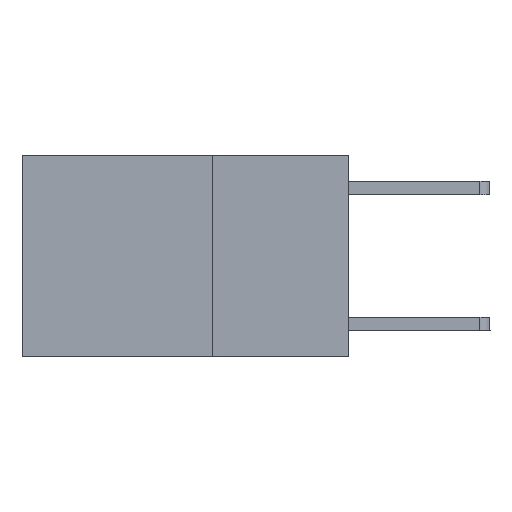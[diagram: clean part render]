
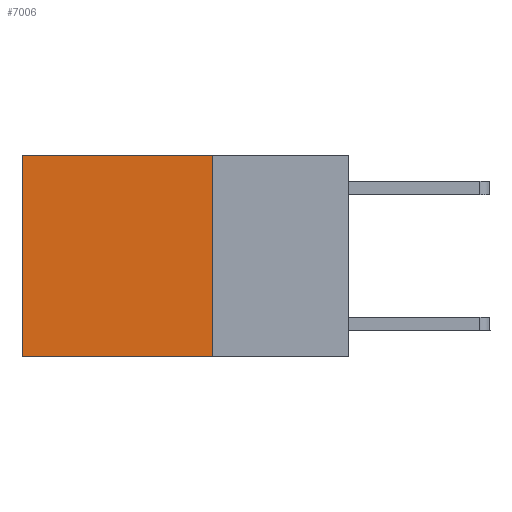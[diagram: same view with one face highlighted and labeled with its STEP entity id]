
A CAD part, left-side view. The second image highlights one B-rep face of the part: STEP entity #7006.
In plain terms, the highlighted planar face has unit normal (-1, 0, 0).
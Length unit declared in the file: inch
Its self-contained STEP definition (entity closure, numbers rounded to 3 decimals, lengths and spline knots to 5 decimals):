
#231 = EDGE_CURVE ( 'NONE', #5409, #7527, #5447, .T. ) ;
#343 = EDGE_CURVE ( 'NONE', #8316, #1577, #7993, .T. ) ;
#571 = ORIENTED_EDGE ( 'NONE', *, *, #9104, .T. ) ;
#599 = ORIENTED_EDGE ( 'NONE', *, *, #231, .F. ) ;
#680 = ORIENTED_EDGE ( 'NONE', *, *, #9577, .F. ) ;
#761 = ORIENTED_EDGE ( 'NONE', *, *, #343, .T. ) ;
#1028 = VECTOR ( 'NONE', #2379, 39.37008 ) ;
#1073 = VECTOR ( 'NONE', #7984, 39.37008 ) ;
#1354 = LINE ( 'NONE', #2268, #1073 ) ;
#1577 = VERTEX_POINT ( 'NONE', #9582 ) ;
#1933 = FACE_OUTER_BOUND ( 'NONE', #2931, .T. ) ;
#2268 = CARTESIAN_POINT ( 'NONE',  ( 0.2625, 0.6, 0. ) ) ;
#2379 = DIRECTION ( 'NONE',  ( 0., 1., 0. ) ) ;
#2931 = EDGE_LOOP ( 'NONE', ( #571, #599, #680, #761 ) ) ;
#3829 = VECTOR ( 'NONE', #4377, 39.37008 ) ;
#3864 = CARTESIAN_POINT ( 'NONE',  ( 0.2625, 0.25, -0.37 ) ) ;
#4267 = CARTESIAN_POINT ( 'NONE',  ( 0.2625, 0.25, 0. ) ) ;
#4377 = DIRECTION ( 'NONE',  ( 0., 0., -1. ) ) ;
#4650 = CARTESIAN_POINT ( 'NONE',  ( 0.2625, 0.25, 0. ) ) ;
#5080 = DIRECTION ( 'NONE',  ( 1., 0., 0. ) ) ;
#5409 = VERTEX_POINT ( 'NONE', #8911 ) ;
#5447 = LINE ( 'NONE', #3864, #1028 ) ;
#5826 = VECTOR ( 'NONE', #6041, 39.37008 ) ;
#6041 = DIRECTION ( 'NONE',  ( 0., 1., 0. ) ) ;
#6468 = CARTESIAN_POINT ( 'NONE',  ( 0.2625, 0.6, -0.37 ) ) ;
#6626 = CARTESIAN_POINT ( 'NONE',  ( 0.2625, 0.25, 0. ) ) ;
#7006 = ADVANCED_FACE ( 'NONE', ( #1933 ), #9063, .F. ) ;
#7527 = VERTEX_POINT ( 'NONE', #6468 ) ;
#7911 = LINE ( 'NONE', #8397, #3829 ) ;
#7984 = DIRECTION ( 'NONE',  ( 0., 0., -1. ) ) ;
#7993 = LINE ( 'NONE', #4650, #5826 ) ;
#8316 = VERTEX_POINT ( 'NONE', #6626 ) ;
#8397 = CARTESIAN_POINT ( 'NONE',  ( 0.2625, 0.25, 0. ) ) ;
#8652 = AXIS2_PLACEMENT_3D ( 'NONE', #4267, #5080, #10571 ) ;
#8911 = CARTESIAN_POINT ( 'NONE',  ( 0.2625, 0.25, -0.37 ) ) ;
#9063 = PLANE ( 'NONE',  #8652 ) ;
#9104 = EDGE_CURVE ( 'NONE', #1577, #7527, #1354, .T. ) ;
#9577 = EDGE_CURVE ( 'NONE', #8316, #5409, #7911, .T. ) ;
#9582 = CARTESIAN_POINT ( 'NONE',  ( 0.2625, 0.6, 0. ) ) ;
#10571 = DIRECTION ( 'NONE',  ( 0., 0., -1. ) ) ;
